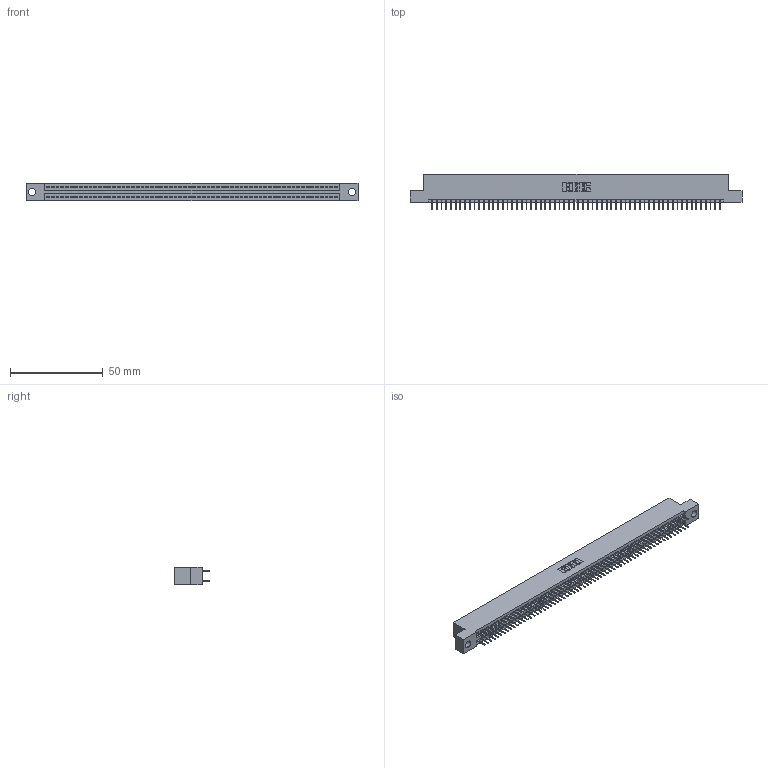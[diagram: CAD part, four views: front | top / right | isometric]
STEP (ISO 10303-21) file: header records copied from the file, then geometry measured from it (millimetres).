
FILE_DESCRIPTION (( 'STEP AP203' ), '1' );
FILE_NAME ('345-124-524-204.STEP', '2021-05-25T18:15:15', ( '' ), ( '' ), 'SwSTEP 2.0', 'SolidWorks 2020', '' );
FILE_SCHEMA (( 'CONFIG_CONTROL_DESIGN' ));
Length unit declared in the file: inch
Products named in the file (3): 345 Part_Flush Mounting Lugs - 0.156 Dia-TI; 345-292-001_345-293-124; 345-124-524-204
Assembly tree (125 placements, depth 2):
  345-124-524-204
    345 Part_Flush Mounting Lugs - 0.156 Dia-TI
    345-292-001_345-293-124  x124
Bounding box: 178.69 x 19.35 x 9.4 mm (x, y, z)
Volume: 17250.1 mm3; surface area: 25242.1 mm2
Topology: 125 solids, 125 shells, 6836 faces, 19349 edges, 12402 vertices
Faces by surface type: plane 4930, cylinder 1906
Entity records: 46447 total; most frequent: CARTESIAN_POINT 7770, ORIENTED_EDGE 7702, DIRECTION 6827, EDGE_CURVE 3851, VECTOR 3475, LINE 3475, VERTEX_POINT 2562, AXIS2_PLACEMENT_3D 1676
